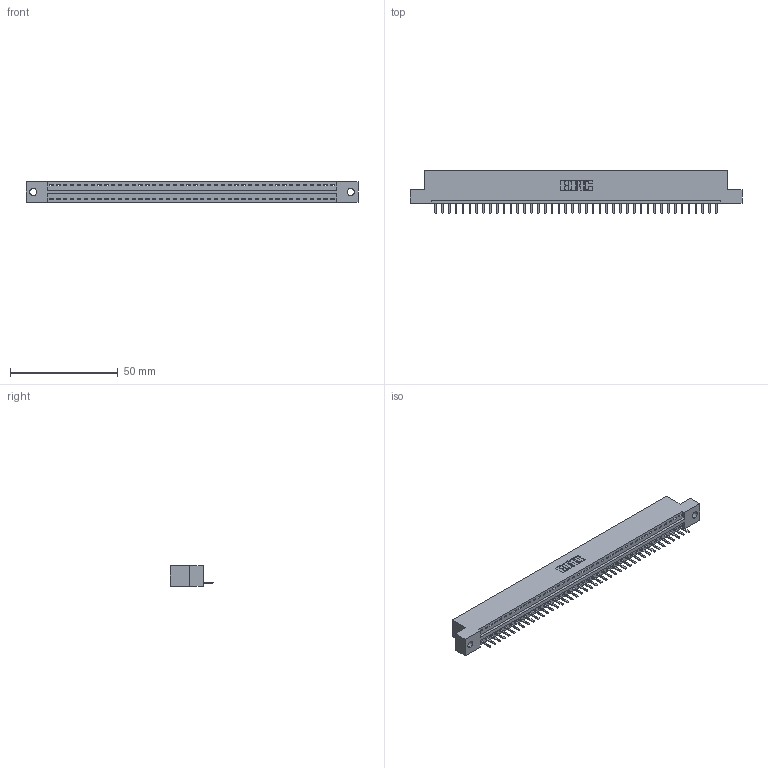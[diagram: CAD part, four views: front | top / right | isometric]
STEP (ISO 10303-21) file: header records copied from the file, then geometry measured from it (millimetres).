
FILE_DESCRIPTION (( 'STEP AP203' ), '1' );
FILE_NAME ('346-042-520-102.STEP', '2022-05-09T14:01:04', ( '' ), ( '' ), 'SwSTEP 2.0', 'SolidWorks 2020', '' );
FILE_SCHEMA (( 'CONFIG_CONTROL_DESIGN' ));
Length unit declared in the file: inch
Products named in the file (3): 346 Part_Flush Mounting Lugs - 0.128 Dia; 345-292-001_345-293-120; 346-042-520-102
Assembly tree (43 placements, depth 2):
  346-042-520-102
    346 Part_Flush Mounting Lugs - 0.128 Dia
    345-292-001_345-293-120  x42
Bounding box: 153.92 x 20.02 x 9.4 mm (x, y, z)
Volume: 14576.4 mm3; surface area: 17544.1 mm2
Topology: 43 solids, 43 shells, 2726 faces, 8057 edges, 5258 vertices
Faces by surface type: plane 1840, cylinder 886
Entity records: 26183 total; most frequent: CARTESIAN_POINT 4506, ORIENTED_EDGE 4470, DIRECTION 3963, EDGE_CURVE 2235, VECTOR 1931, LINE 1931, VERTEX_POINT 1486, AXIS2_PLACEMENT_3D 1016
